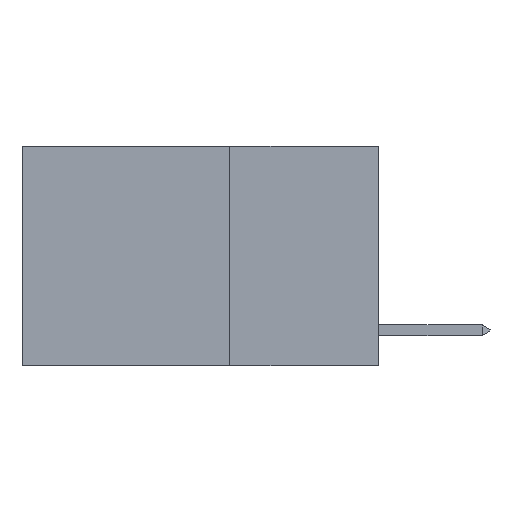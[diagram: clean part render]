
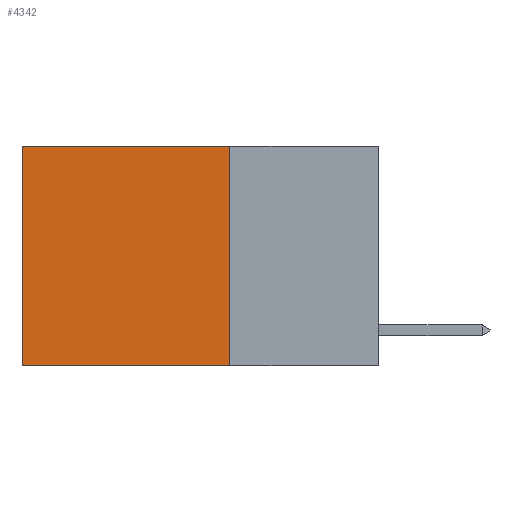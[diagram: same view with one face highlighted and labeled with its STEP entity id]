
A CAD part, left-side view. The second image highlights one B-rep face of the part: STEP entity #4342.
In plain terms, the highlighted planar face has unit normal (-1, 0, 0).
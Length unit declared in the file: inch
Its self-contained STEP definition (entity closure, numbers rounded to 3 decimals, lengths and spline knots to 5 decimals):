
#349 = DIRECTION ( 'NONE',  ( 0., 0., -1. ) ) ;
#411 = DIRECTION ( 'NONE',  ( 1., 0., 0. ) ) ;
#583 = PLANE ( 'NONE',  #9311 ) ;
#937 = CARTESIAN_POINT ( 'NONE',  ( 0.2625, 0.25, 0. ) ) ;
#956 = CARTESIAN_POINT ( 'NONE',  ( 0.2625, 0.25, 0. ) ) ;
#964 = DIRECTION ( 'NONE',  ( 0., 0., -1. ) ) ;
#1094 = LINE ( 'NONE', #3454, #9415 ) ;
#1543 = CARTESIAN_POINT ( 'NONE',  ( 0.2625, 0.6, -0.37 ) ) ;
#1951 = VERTEX_POINT ( 'NONE', #7361 ) ;
#2217 = VECTOR ( 'NONE', #964, 39.37008 ) ;
#2222 = EDGE_CURVE ( 'NONE', #3346, #1951, #7666, .T. ) ;
#3346 = VERTEX_POINT ( 'NONE', #7512 ) ;
#3454 = CARTESIAN_POINT ( 'NONE',  ( 0.2625, 0.6, 0. ) ) ;
#3695 = CARTESIAN_POINT ( 'NONE',  ( 0.2625, 0.25, -0.37 ) ) ;
#4159 = EDGE_CURVE ( 'NONE', #3346, #9207, #8398, .T. ) ;
#4168 = DIRECTION ( 'NONE',  ( 0., 1., 0. ) ) ;
#4342 = ADVANCED_FACE ( 'NONE', ( #7255 ), #583, .F. ) ;
#4384 = CARTESIAN_POINT ( 'NONE',  ( 0.2625, 0.25, 0. ) ) ;
#4399 = EDGE_LOOP ( 'NONE', ( #8620, #8636, #8655, #8666 ) ) ;
#4585 = DIRECTION ( 'NONE',  ( 0., 1., 0. ) ) ;
#4664 = EDGE_CURVE ( 'NONE', #9207, #5911, #7248, .T. ) ;
#5911 = VERTEX_POINT ( 'NONE', #1543 ) ;
#7248 = LINE ( 'NONE', #3695, #9120 ) ;
#7255 = FACE_OUTER_BOUND ( 'NONE', #4399, .T. ) ;
#7286 = EDGE_CURVE ( 'NONE', #1951, #5911, #1094, .T. ) ;
#7361 = CARTESIAN_POINT ( 'NONE',  ( 0.2625, 0.6, 0. ) ) ;
#7416 = VECTOR ( 'NONE', #4168, 39.37008 ) ;
#7512 = CARTESIAN_POINT ( 'NONE',  ( 0.2625, 0.25, 0. ) ) ;
#7666 = LINE ( 'NONE', #4384, #7416 ) ;
#8398 = LINE ( 'NONE', #937, #2217 ) ;
#8530 = DIRECTION ( 'NONE',  ( 0., 0., -1. ) ) ;
#8620 = ORIENTED_EDGE ( 'NONE', *, *, #7286, .T. ) ;
#8636 = ORIENTED_EDGE ( 'NONE', *, *, #4664, .F. ) ;
#8655 = ORIENTED_EDGE ( 'NONE', *, *, #4159, .F. ) ;
#8666 = ORIENTED_EDGE ( 'NONE', *, *, #2222, .T. ) ;
#9120 = VECTOR ( 'NONE', #4585, 39.37008 ) ;
#9207 = VERTEX_POINT ( 'NONE', #9660 ) ;
#9311 = AXIS2_PLACEMENT_3D ( 'NONE', #956, #411, #349 ) ;
#9415 = VECTOR ( 'NONE', #8530, 39.37008 ) ;
#9660 = CARTESIAN_POINT ( 'NONE',  ( 0.2625, 0.25, -0.37 ) ) ;
